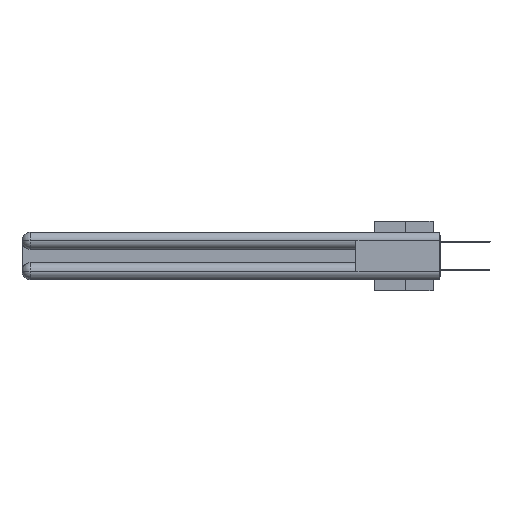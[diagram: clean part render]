
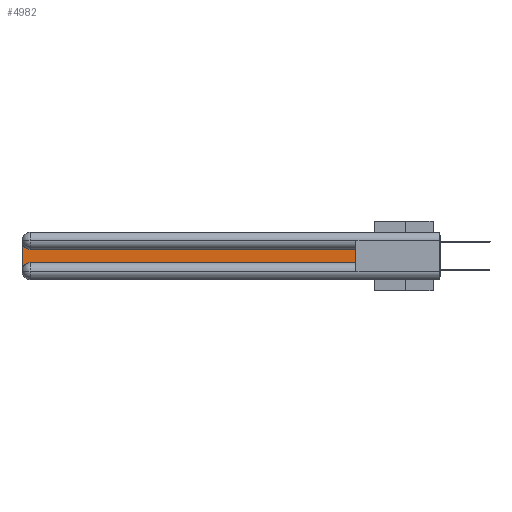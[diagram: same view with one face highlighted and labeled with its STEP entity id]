
A CAD part, left-side view. The second image highlights one B-rep face of the part: STEP entity #4982.
In plain terms, the highlighted planar face has unit normal (-1, 0, 0).
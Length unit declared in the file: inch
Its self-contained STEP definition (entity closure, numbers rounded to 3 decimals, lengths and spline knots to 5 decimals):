
#34 = VECTOR ( 'NONE', #3737, 39.37008 ) ;
#99 = ORIENTED_EDGE ( 'NONE', *, *, #22295, .T. ) ;
#1094 = CARTESIAN_POINT ( 'NONE',  ( 0.075, 0.6, -0.1225 ) ) ;
#1332 = DIRECTION ( 'NONE',  ( 1., 0., 0. ) ) ;
#1544 = DIRECTION ( 'NONE',  ( 0., 0., -1. ) ) ;
#2022 = VECTOR ( 'NONE', #28019, 39.37008 ) ;
#2681 = CARTESIAN_POINT ( 'NONE',  ( 0.075, 0.6, -0.1225 ) ) ;
#3235 = CARTESIAN_POINT ( 'NONE',  ( 0.075, 0.6, -0.2175 ) ) ;
#3381 = ORIENTED_EDGE ( 'NONE', *, *, #21026, .T. ) ;
#3737 = DIRECTION ( 'NONE',  ( 0., 0., 1. ) ) ;
#4982 = ADVANCED_FACE ( 'NONE', ( #14665 ), #17780, .F. ) ;
#5540 = CARTESIAN_POINT ( 'NONE',  ( 0.075, 3., -0.2775 ) ) ;
#5942 = ORIENTED_EDGE ( 'NONE', *, *, #28139, .T. ) ;
#7457 = EDGE_CURVE ( 'NONE', #19273, #19776, #29769, .T. ) ;
#7735 = VERTEX_POINT ( 'NONE', #14174 ) ;
#10200 = EDGE_CURVE ( 'NONE', #19776, #7735, #14392, .T. ) ;
#10827 = VECTOR ( 'NONE', #26292, 39.37008 ) ;
#11070 = VERTEX_POINT ( 'NONE', #5540 ) ;
#12617 = AXIS2_PLACEMENT_3D ( 'NONE', #12830, #1332, #12932 ) ;
#12830 = CARTESIAN_POINT ( 'NONE',  ( 0.075, 3., -0.1225 ) ) ;
#12868 = CARTESIAN_POINT ( 'NONE',  ( 0.075, 2.94, -0.0625 ) ) ;
#12932 = DIRECTION ( 'NONE',  ( 0., 0., -1. ) ) ;
#13214 = CARTESIAN_POINT ( 'NONE',  ( 0.075, 0.6, -0.2175 ) ) ;
#14174 = CARTESIAN_POINT ( 'NONE',  ( 0.075, 2.94, -0.1225 ) ) ;
#14392 = LINE ( 'NONE', #2681, #2022 ) ;
#14665 = FACE_OUTER_BOUND ( 'NONE', #17705, .T. ) ;
#15444 = DIRECTION ( 'NONE',  ( 1., 0., 0. ) ) ;
#16961 = LINE ( 'NONE', #26189, #10827 ) ;
#17705 = EDGE_LOOP ( 'NONE', ( #17986, #3381, #5942, #24840, #99, #28484 ) ) ;
#17780 = PLANE ( 'NONE',  #12617 ) ;
#17986 = ORIENTED_EDGE ( 'NONE', *, *, #10200, .T. ) ;
#18949 = AXIS2_PLACEMENT_3D ( 'NONE', #12868, #24583, #26900 ) ;
#19273 = VERTEX_POINT ( 'NONE', #20282 ) ;
#19776 = VERTEX_POINT ( 'NONE', #1094 ) ;
#19784 = DIRECTION ( 'NONE',  ( 0., -1., 0. ) ) ;
#19960 = VECTOR ( 'NONE', #19784, 39.37008 ) ;
#20197 = CARTESIAN_POINT ( 'NONE',  ( 0.075, 2.94, -0.2775 ) ) ;
#20282 = CARTESIAN_POINT ( 'NONE',  ( 0.075, 0.6, -0.2175 ) ) ;
#21026 = EDGE_CURVE ( 'NONE', #7735, #21947, #24010, .T. ) ;
#21947 = VERTEX_POINT ( 'NONE', #25937 ) ;
#22295 = EDGE_CURVE ( 'NONE', #29511, #19273, #26079, .T. ) ;
#24010 = CIRCLE ( 'NONE', #18949, 0.06 ) ;
#24583 = DIRECTION ( 'NONE',  ( 1., 0., 0. ) ) ;
#24840 = ORIENTED_EDGE ( 'NONE', *, *, #27079, .T. ) ;
#25937 = CARTESIAN_POINT ( 'NONE',  ( 0.075, 3., -0.0625 ) ) ;
#26079 = LINE ( 'NONE', #13214, #19960 ) ;
#26189 = CARTESIAN_POINT ( 'NONE',  ( 0.075, 3., -0.2175 ) ) ;
#26292 = DIRECTION ( 'NONE',  ( 0., 0., -1. ) ) ;
#26900 = DIRECTION ( 'NONE',  ( 0., 0., -1. ) ) ;
#27079 = EDGE_CURVE ( 'NONE', #11070, #29511, #27893, .T. ) ;
#27181 = AXIS2_PLACEMENT_3D ( 'NONE', #20197, #15444, #1544 ) ;
#27893 = CIRCLE ( 'NONE', #27181, 0.06 ) ;
#28019 = DIRECTION ( 'NONE',  ( 0., 1., 0. ) ) ;
#28139 = EDGE_CURVE ( 'NONE', #21947, #11070, #16961, .T. ) ;
#28484 = ORIENTED_EDGE ( 'NONE', *, *, #7457, .T. ) ;
#28967 = CARTESIAN_POINT ( 'NONE',  ( 0.075, 2.94, -0.2175 ) ) ;
#29511 = VERTEX_POINT ( 'NONE', #28967 ) ;
#29769 = LINE ( 'NONE', #3235, #34 ) ;
